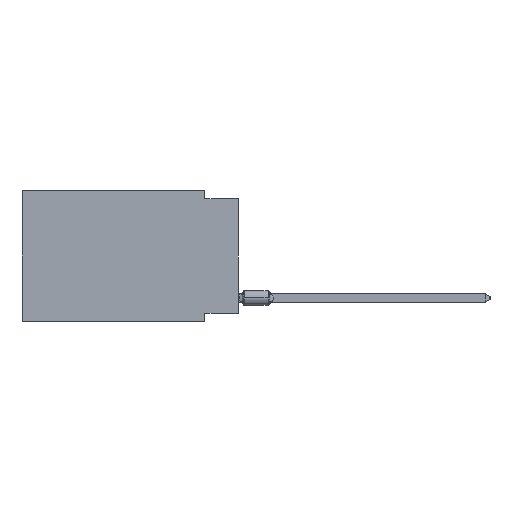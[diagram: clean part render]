
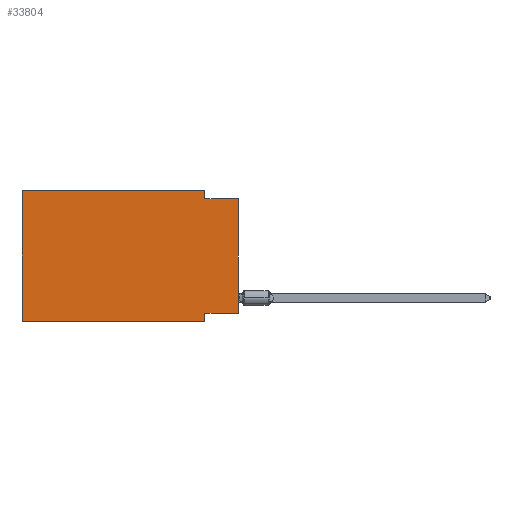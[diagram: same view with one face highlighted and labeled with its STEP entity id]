
A CAD part, left-side view. The second image highlights one B-rep face of the part: STEP entity #33804.
In plain terms, the highlighted planar face has unit normal (-1, 0, 0).
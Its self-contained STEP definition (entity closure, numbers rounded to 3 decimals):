
#472 = DIRECTION ( 'NONE',  ( 0., -1., 0. ) ) ;
#1000 = LINE ( 'NONE', #20709, #40412 ) ;
#1338 = ORIENTED_EDGE ( 'NONE', *, *, #23095, .F. ) ;
#1919 = VERTEX_POINT ( 'NONE', #2112 ) ;
#2112 = CARTESIAN_POINT ( 'NONE',  ( 0., 2.54, -9.271 ) ) ;
#2594 = EDGE_CURVE ( 'NONE', #50172, #2912, #41758, .T. ) ;
#2912 = VERTEX_POINT ( 'NONE', #35999 ) ;
#3720 = DIRECTION ( 'NONE',  ( 0., 0., -1. ) ) ;
#5552 = EDGE_CURVE ( 'NONE', #50172, #44550, #30830, .T. ) ;
#5591 = DIRECTION ( 'NONE',  ( 0., -1., 0. ) ) ;
#5777 = LINE ( 'NONE', #33631, #23678 ) ;
#6887 = ORIENTED_EDGE ( 'NONE', *, *, #23945, .F. ) ;
#7351 = LINE ( 'NONE', #27264, #10499 ) ;
#9023 = ORIENTED_EDGE ( 'NONE', *, *, #42783, .F. ) ;
#9335 = ORIENTED_EDGE ( 'NONE', *, *, #26207, .T. ) ;
#10386 = CARTESIAN_POINT ( 'NONE',  ( 0., 16.383, 0. ) ) ;
#10499 = VECTOR ( 'NONE', #10539, 1000. ) ;
#10539 = DIRECTION ( 'NONE',  ( 0., 0., 1. ) ) ;
#10731 = DIRECTION ( 'NONE',  ( 0., 0., -1. ) ) ;
#11195 = VECTOR ( 'NONE', #10731, 1000. ) ;
#11371 = CARTESIAN_POINT ( 'NONE',  ( 0., 0., -9.271 ) ) ;
#11965 = ORIENTED_EDGE ( 'NONE', *, *, #5552, .T. ) ;
#12286 = VECTOR ( 'NONE', #46001, 1000. ) ;
#14087 = PLANE ( 'NONE',  #15944 ) ;
#14357 = DIRECTION ( 'NONE',  ( 1., 0., 0. ) ) ;
#14613 = LINE ( 'NONE', #38761, #15346 ) ;
#15346 = VECTOR ( 'NONE', #34788, 1000. ) ;
#15944 = AXIS2_PLACEMENT_3D ( 'NONE', #10386, #14357, #3720 ) ;
#17617 = CARTESIAN_POINT ( 'NONE',  ( 0., 16.383, 0. ) ) ;
#18349 = ORIENTED_EDGE ( 'NONE', *, *, #32689, .F. ) ;
#20709 = CARTESIAN_POINT ( 'NONE',  ( 0., 16.383, 0. ) ) ;
#22547 = CARTESIAN_POINT ( 'NONE',  ( 0., 16.383, -9.906 ) ) ;
#23095 = EDGE_CURVE ( 'NONE', #50252, #1919, #5777, .T. ) ;
#23176 = CARTESIAN_POINT ( 'NONE',  ( 0., 2.54, -0.635 ) ) ;
#23678 = VECTOR ( 'NONE', #41861, 1000. ) ;
#23945 = EDGE_CURVE ( 'NONE', #30698, #42234, #14613, .T. ) ;
#25482 = DIRECTION ( 'NONE',  ( 0., 0., -1. ) ) ;
#26207 = EDGE_CURVE ( 'NONE', #50252, #42234, #7351, .T. ) ;
#26895 = EDGE_LOOP ( 'NONE', ( #9335, #6887, #9023, #18349, #43997, #11965, #35623, #1338 ) ) ;
#27264 = CARTESIAN_POINT ( 'NONE',  ( 0., 0., 0. ) ) ;
#30646 = CARTESIAN_POINT ( 'NONE',  ( 0., 2.54, -9.906 ) ) ;
#30698 = VERTEX_POINT ( 'NONE', #23176 ) ;
#30830 = LINE ( 'NONE', #42748, #41361 ) ;
#31086 = CARTESIAN_POINT ( 'NONE',  ( 0., 2.54, -9.906 ) ) ;
#32689 = EDGE_CURVE ( 'NONE', #2912, #47855, #1000, .T. ) ;
#33631 = CARTESIAN_POINT ( 'NONE',  ( 0., 0., -9.271 ) ) ;
#33804 = ADVANCED_FACE ( 'NONE', ( #34534 ), #14087, .F. ) ;
#34074 = VECTOR ( 'NONE', #25482, 1000. ) ;
#34505 = LINE ( 'NONE', #50664, #34074 ) ;
#34534 = FACE_OUTER_BOUND ( 'NONE', #26895, .T. ) ;
#34788 = DIRECTION ( 'NONE',  ( 0., -1., 0. ) ) ;
#35623 = ORIENTED_EDGE ( 'NONE', *, *, #36516, .F. ) ;
#35999 = CARTESIAN_POINT ( 'NONE',  ( 0., 16.383, 0. ) ) ;
#36220 = CARTESIAN_POINT ( 'NONE',  ( 0., 2.54, 0. ) ) ;
#36516 = EDGE_CURVE ( 'NONE', #1919, #44550, #50775, .T. ) ;
#38761 = CARTESIAN_POINT ( 'NONE',  ( 0., 0., -0.635 ) ) ;
#40412 = VECTOR ( 'NONE', #472, 1000. ) ;
#41361 = VECTOR ( 'NONE', #5591, 1000. ) ;
#41758 = LINE ( 'NONE', #17617, #12286 ) ;
#41861 = DIRECTION ( 'NONE',  ( 0., 1., 0. ) ) ;
#42234 = VERTEX_POINT ( 'NONE', #47312 ) ;
#42748 = CARTESIAN_POINT ( 'NONE',  ( 0., 16.383, -9.906 ) ) ;
#42783 = EDGE_CURVE ( 'NONE', #47855, #30698, #34505, .T. ) ;
#43997 = ORIENTED_EDGE ( 'NONE', *, *, #2594, .F. ) ;
#44550 = VERTEX_POINT ( 'NONE', #31086 ) ;
#46001 = DIRECTION ( 'NONE',  ( 0., 0., 1. ) ) ;
#47312 = CARTESIAN_POINT ( 'NONE',  ( 0., 0., -0.635 ) ) ;
#47855 = VERTEX_POINT ( 'NONE', #36220 ) ;
#50172 = VERTEX_POINT ( 'NONE', #22547 ) ;
#50252 = VERTEX_POINT ( 'NONE', #11371 ) ;
#50664 = CARTESIAN_POINT ( 'NONE',  ( 0., 2.54, 0. ) ) ;
#50775 = LINE ( 'NONE', #30646, #11195 ) ;
